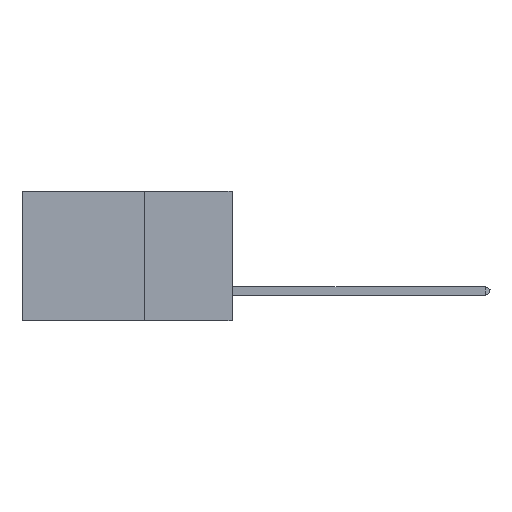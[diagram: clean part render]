
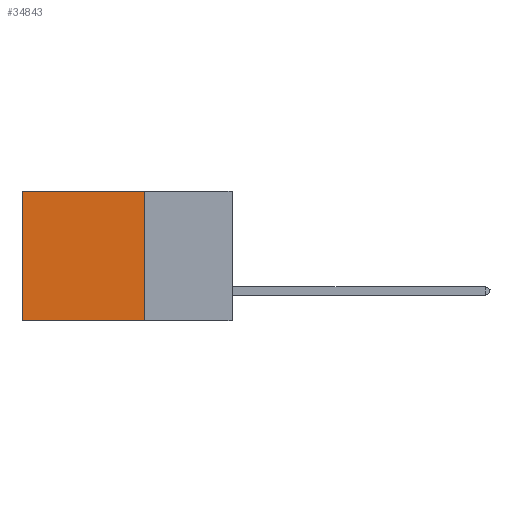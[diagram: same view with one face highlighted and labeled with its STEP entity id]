
A CAD part, left-side view. The second image highlights one B-rep face of the part: STEP entity #34843.
In plain terms, the highlighted planar face has unit normal (-1, 0, 0).
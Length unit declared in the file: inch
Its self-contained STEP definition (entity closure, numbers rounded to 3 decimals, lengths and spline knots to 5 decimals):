
#2293 = VERTEX_POINT ( 'NONE', #16828 ) ;
#4101 = LINE ( 'NONE', #39822, #22534 ) ;
#4555 = LINE ( 'NONE', #39064, #13862 ) ;
#6376 = CARTESIAN_POINT ( 'NONE',  ( 0.2875, 0.6, -0.37 ) ) ;
#6818 = VECTOR ( 'NONE', #34256, 39.37008 ) ;
#7980 = DIRECTION ( 'NONE',  ( 0., 0., -1. ) ) ;
#10482 = EDGE_CURVE ( 'NONE', #31349, #44942, #16066, .T. ) ;
#10947 = EDGE_CURVE ( 'NONE', #44942, #25349, #4555, .T. ) ;
#11310 = LINE ( 'NONE', #38326, #42268 ) ;
#12381 = ORIENTED_EDGE ( 'NONE', *, *, #10482, .F. ) ;
#13862 = VECTOR ( 'NONE', #24733, 39.37008 ) ;
#14397 = CARTESIAN_POINT ( 'NONE',  ( 0.2875, 0.25, 0. ) ) ;
#16066 = LINE ( 'NONE', #23743, #6818 ) ;
#16828 = CARTESIAN_POINT ( 'NONE',  ( 0.2875, 0.6, 0. ) ) ;
#17345 = EDGE_LOOP ( 'NONE', ( #24195, #28275, #12381, #40953 ) ) ;
#17644 = FACE_OUTER_BOUND ( 'NONE', #17345, .T. ) ;
#17985 = CARTESIAN_POINT ( 'NONE',  ( 0.2875, 0.25, -0.37 ) ) ;
#22534 = VECTOR ( 'NONE', #28771, 39.37008 ) ;
#23743 = CARTESIAN_POINT ( 'NONE',  ( 0.2875, 0.25, 0. ) ) ;
#24195 = ORIENTED_EDGE ( 'NONE', *, *, #40509, .T. ) ;
#24733 = DIRECTION ( 'NONE',  ( 0., 1., 0. ) ) ;
#25349 = VERTEX_POINT ( 'NONE', #6376 ) ;
#27128 = AXIS2_PLACEMENT_3D ( 'NONE', #14397, #29032, #7980 ) ;
#27276 = CARTESIAN_POINT ( 'NONE',  ( 0.2875, 0.25, 0. ) ) ;
#28107 = PLANE ( 'NONE',  #27128 ) ;
#28275 = ORIENTED_EDGE ( 'NONE', *, *, #10947, .F. ) ;
#28771 = DIRECTION ( 'NONE',  ( 0., 0., -1. ) ) ;
#29032 = DIRECTION ( 'NONE',  ( 1., 0., 0. ) ) ;
#31349 = VERTEX_POINT ( 'NONE', #27276 ) ;
#34256 = DIRECTION ( 'NONE',  ( 0., 0., -1. ) ) ;
#34843 = ADVANCED_FACE ( 'NONE', ( #17644 ), #28107, .F. ) ;
#38208 = EDGE_CURVE ( 'NONE', #31349, #2293, #11310, .T. ) ;
#38326 = CARTESIAN_POINT ( 'NONE',  ( 0.2875, 0.25, 0. ) ) ;
#39064 = CARTESIAN_POINT ( 'NONE',  ( 0.2875, 0.25, -0.37 ) ) ;
#39822 = CARTESIAN_POINT ( 'NONE',  ( 0.2875, 0.6, 0. ) ) ;
#40509 = EDGE_CURVE ( 'NONE', #2293, #25349, #4101, .T. ) ;
#40953 = ORIENTED_EDGE ( 'NONE', *, *, #38208, .T. ) ;
#41824 = DIRECTION ( 'NONE',  ( 0., 1., 0. ) ) ;
#42268 = VECTOR ( 'NONE', #41824, 39.37008 ) ;
#44942 = VERTEX_POINT ( 'NONE', #17985 ) ;
